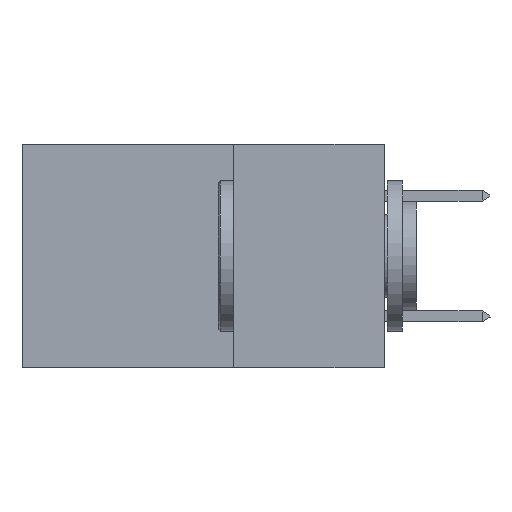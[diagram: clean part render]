
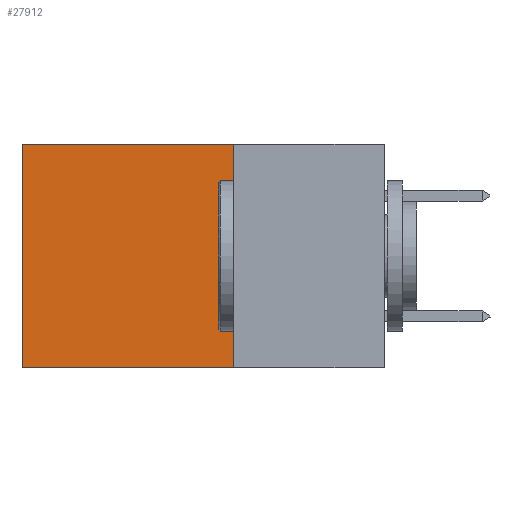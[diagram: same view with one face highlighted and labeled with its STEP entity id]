
A CAD part, left-side view. The second image highlights one B-rep face of the part: STEP entity #27912.
In plain terms, the highlighted planar face has unit normal (-1, 0, 0).
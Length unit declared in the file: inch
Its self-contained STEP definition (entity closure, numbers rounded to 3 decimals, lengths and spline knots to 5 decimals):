
#764 = DIRECTION ( 'NONE',  ( 0., 0., -1. ) ) ;
#1362 = DIRECTION ( 'NONE',  ( 0., 1., 0. ) ) ;
#2491 = EDGE_LOOP ( 'NONE', ( #5674, #18465, #22858, #7295 ) ) ;
#3228 = VERTEX_POINT ( 'NONE', #15938 ) ;
#3582 = DIRECTION ( 'NONE',  ( 0., 1., 0. ) ) ;
#4219 = VERTEX_POINT ( 'NONE', #6930 ) ;
#4857 = CARTESIAN_POINT ( 'NONE',  ( 0.2875, 0.25, 0. ) ) ;
#5674 = ORIENTED_EDGE ( 'NONE', *, *, #8026, .T. ) ;
#6930 = CARTESIAN_POINT ( 'NONE',  ( 0.2875, 0.6, 0. ) ) ;
#7295 = ORIENTED_EDGE ( 'NONE', *, *, #12759, .T. ) ;
#7860 = CARTESIAN_POINT ( 'NONE',  ( 0.2875, 0.25, -0.37 ) ) ;
#8026 = EDGE_CURVE ( 'NONE', #4219, #21653, #26124, .T. ) ;
#9012 = CARTESIAN_POINT ( 'NONE',  ( 0.2875, 0.6, -0.37 ) ) ;
#9872 = CARTESIAN_POINT ( 'NONE',  ( 0.2875, 0.25, 0. ) ) ;
#11028 = EDGE_CURVE ( 'NONE', #17146, #3228, #25987, .T. ) ;
#12739 = CARTESIAN_POINT ( 'NONE',  ( 0.2875, 0.25, 0. ) ) ;
#12759 = EDGE_CURVE ( 'NONE', #17146, #4219, #18366, .T. ) ;
#13517 = DIRECTION ( 'NONE',  ( 0., 0., -1. ) ) ;
#13850 = LINE ( 'NONE', #7860, #14542 ) ;
#13869 = VECTOR ( 'NONE', #3582, 39.37008 ) ;
#14430 = PLANE ( 'NONE',  #19892 ) ;
#14542 = VECTOR ( 'NONE', #1362, 39.37008 ) ;
#15938 = CARTESIAN_POINT ( 'NONE',  ( 0.2875, 0.25, -0.37 ) ) ;
#16678 = CARTESIAN_POINT ( 'NONE',  ( 0.2875, 0.6, 0. ) ) ;
#17146 = VERTEX_POINT ( 'NONE', #21094 ) ;
#18366 = LINE ( 'NONE', #12739, #13869 ) ;
#18465 = ORIENTED_EDGE ( 'NONE', *, *, #24423, .F. ) ;
#18593 = DIRECTION ( 'NONE',  ( 1., 0., 0. ) ) ;
#19892 = AXIS2_PLACEMENT_3D ( 'NONE', #9872, #18593, #764 ) ;
#20595 = FACE_OUTER_BOUND ( 'NONE', #2491, .T. ) ;
#21094 = CARTESIAN_POINT ( 'NONE',  ( 0.2875, 0.25, 0. ) ) ;
#21117 = DIRECTION ( 'NONE',  ( 0., 0., -1. ) ) ;
#21306 = VECTOR ( 'NONE', #21117, 39.37008 ) ;
#21653 = VERTEX_POINT ( 'NONE', #9012 ) ;
#22858 = ORIENTED_EDGE ( 'NONE', *, *, #11028, .F. ) ;
#24423 = EDGE_CURVE ( 'NONE', #3228, #21653, #13850, .T. ) ;
#25987 = LINE ( 'NONE', #4857, #28737 ) ;
#26124 = LINE ( 'NONE', #16678, #21306 ) ;
#27912 = ADVANCED_FACE ( 'NONE', ( #20595 ), #14430, .F. ) ;
#28737 = VECTOR ( 'NONE', #13517, 39.37008 ) ;
